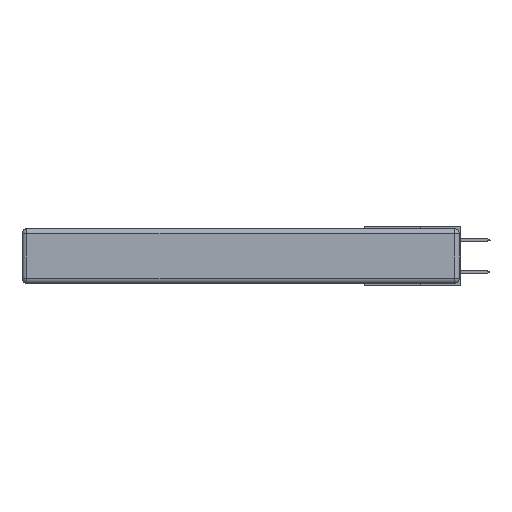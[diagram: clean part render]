
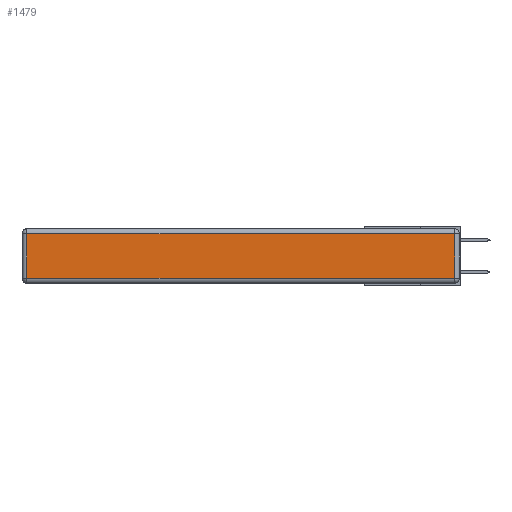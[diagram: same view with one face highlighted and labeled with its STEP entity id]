
A CAD part, left-side view. The second image highlights one B-rep face of the part: STEP entity #1479.
In plain terms, the highlighted planar face has unit normal (-1, 0, 0).
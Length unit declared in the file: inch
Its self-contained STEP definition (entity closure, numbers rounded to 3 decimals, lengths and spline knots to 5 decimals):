
#923 = EDGE_CURVE ( 'NONE', #24610, #21962, #14091, .T. ) ;
#1479 = ADVANCED_FACE ( 'NONE', ( #3811 ), #24110, .T. ) ;
#1495 = ORIENTED_EDGE ( 'NONE', *, *, #7753, .T. ) ;
#1520 = VECTOR ( 'NONE', #14664, 39.37008 ) ;
#2860 = VECTOR ( 'NONE', #9019, 39.37008 ) ;
#3811 = FACE_OUTER_BOUND ( 'NONE', #18618, .T. ) ;
#3871 = LINE ( 'NONE', #24375, #15581 ) ;
#4428 = ORIENTED_EDGE ( 'NONE', *, *, #9897, .T. ) ;
#7753 = EDGE_CURVE ( 'NONE', #8166, #24610, #21970, .T. ) ;
#8056 = CARTESIAN_POINT ( 'NONE',  ( 0., 0., -0.343 ) ) ;
#8166 = VERTEX_POINT ( 'NONE', #12752 ) ;
#8250 = VECTOR ( 'NONE', #26784, 39.37008 ) ;
#8360 = ORIENTED_EDGE ( 'NONE', *, *, #25745, .T. ) ;
#9019 = DIRECTION ( 'NONE',  ( 0., 0., -1. ) ) ;
#9897 = EDGE_CURVE ( 'NONE', #21962, #15092, #3871, .T. ) ;
#10215 = DIRECTION ( 'NONE',  ( -1., 0., 0. ) ) ;
#10345 = CARTESIAN_POINT ( 'NONE',  ( 0., 0.03, -0.343 ) ) ;
#10473 = DIRECTION ( 'NONE',  ( 0., 1., 0. ) ) ;
#12170 = AXIS2_PLACEMENT_3D ( 'NONE', #8056, #10215, #12957 ) ;
#12752 = CARTESIAN_POINT ( 'NONE',  ( 0., 2.72, -0.313 ) ) ;
#12957 = DIRECTION ( 'NONE',  ( 0., 0., 1. ) ) ;
#13679 = CARTESIAN_POINT ( 'NONE',  ( 0., 0.03, -0.03 ) ) ;
#14091 = LINE ( 'NONE', #10345, #8250 ) ;
#14664 = DIRECTION ( 'NONE',  ( 0., -1., 0. ) ) ;
#15092 = VERTEX_POINT ( 'NONE', #24118 ) ;
#15581 = VECTOR ( 'NONE', #10473, 39.37008 ) ;
#17106 = CARTESIAN_POINT ( 'NONE',  ( 0., 0., -0.313 ) ) ;
#18618 = EDGE_LOOP ( 'NONE', ( #1495, #28737, #4428, #8360 ) ) ;
#21962 = VERTEX_POINT ( 'NONE', #13679 ) ;
#21970 = LINE ( 'NONE', #17106, #1520 ) ;
#24110 = PLANE ( 'NONE',  #12170 ) ;
#24118 = CARTESIAN_POINT ( 'NONE',  ( 0., 2.72, -0.03 ) ) ;
#24375 = CARTESIAN_POINT ( 'NONE',  ( 0., 2.75, -0.03 ) ) ;
#24610 = VERTEX_POINT ( 'NONE', #28496 ) ;
#25745 = EDGE_CURVE ( 'NONE', #15092, #8166, #26972, .T. ) ;
#26784 = DIRECTION ( 'NONE',  ( 0., 0., 1. ) ) ;
#26972 = LINE ( 'NONE', #27355, #2860 ) ;
#27355 = CARTESIAN_POINT ( 'NONE',  ( 0., 2.72, -0.343 ) ) ;
#28496 = CARTESIAN_POINT ( 'NONE',  ( 0., 0.03, -0.313 ) ) ;
#28737 = ORIENTED_EDGE ( 'NONE', *, *, #923, .T. ) ;
